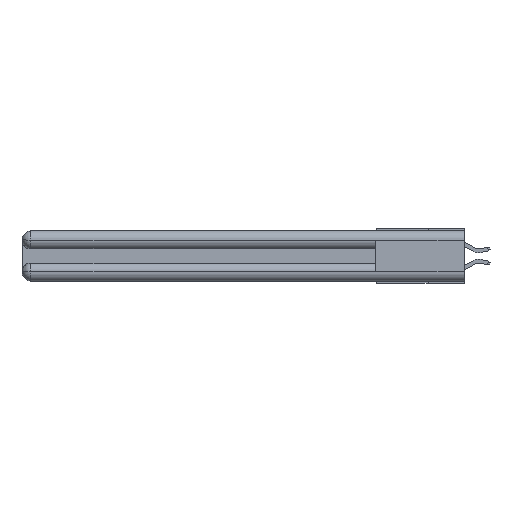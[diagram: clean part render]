
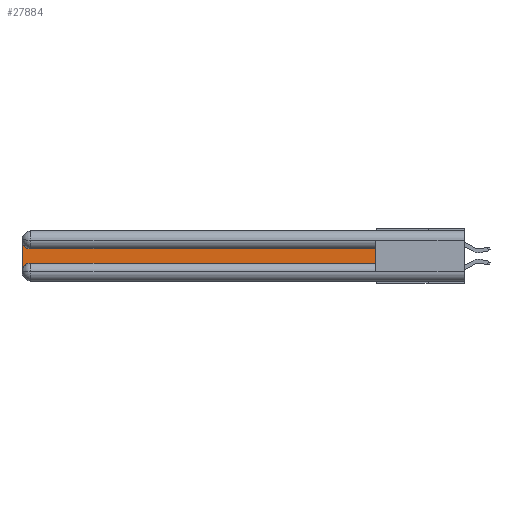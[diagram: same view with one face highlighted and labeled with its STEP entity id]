
A CAD part, left-side view. The second image highlights one B-rep face of the part: STEP entity #27884.
In plain terms, the highlighted planar face has unit normal (-1, 0, 0).
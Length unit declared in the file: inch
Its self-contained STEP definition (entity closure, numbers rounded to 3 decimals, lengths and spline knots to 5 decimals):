
#1772 = DIRECTION ( 'NONE',  ( 0., 0., 1. ) ) ;
#1924 = VERTEX_POINT ( 'NONE', #27431 ) ;
#1940 = VECTOR ( 'NONE', #27641, 39.37008 ) ;
#1979 = CARTESIAN_POINT ( 'NONE',  ( 0.075, 2.94, -0.0625 ) ) ;
#2210 = CARTESIAN_POINT ( 'NONE',  ( 0.075, 2.94, -0.2775 ) ) ;
#2376 = LINE ( 'NONE', #8581, #26684 ) ;
#2886 = LINE ( 'NONE', #5890, #18569 ) ;
#3226 = PLANE ( 'NONE',  #24979 ) ;
#3554 = EDGE_CURVE ( 'NONE', #15105, #20113, #2376, .T. ) ;
#4357 = DIRECTION ( 'NONE',  ( 0., 0., -1. ) ) ;
#5227 = EDGE_LOOP ( 'NONE', ( #24357, #29130, #21365, #7912, #17228, #21772 ) ) ;
#5320 = CARTESIAN_POINT ( 'NONE',  ( 0.075, 3., -0.1225 ) ) ;
#5786 = AXIS2_PLACEMENT_3D ( 'NONE', #1979, #19069, #4357 ) ;
#5890 = CARTESIAN_POINT ( 'NONE',  ( 0.075, 0.6, -0.1225 ) ) ;
#6630 = CARTESIAN_POINT ( 'NONE',  ( 0.075, 3., -0.0625 ) ) ;
#7912 = ORIENTED_EDGE ( 'NONE', *, *, #29048, .T. ) ;
#8039 = DIRECTION ( 'NONE',  ( 1., 0., 0. ) ) ;
#8581 = CARTESIAN_POINT ( 'NONE',  ( 0.075, 0.6, -0.2175 ) ) ;
#11619 = DIRECTION ( 'NONE',  ( 1., 0., 0. ) ) ;
#11685 = LINE ( 'NONE', #15958, #17305 ) ;
#13332 = CARTESIAN_POINT ( 'NONE',  ( 0.075, 0.6, -0.2175 ) ) ;
#14186 = DIRECTION ( 'NONE',  ( 0., 0., -1. ) ) ;
#14983 = DIRECTION ( 'NONE',  ( 0., 1., 0. ) ) ;
#15105 = VERTEX_POINT ( 'NONE', #16944 ) ;
#15958 = CARTESIAN_POINT ( 'NONE',  ( 0.075, 3., -0.2175 ) ) ;
#16944 = CARTESIAN_POINT ( 'NONE',  ( 0.075, 0.6, -0.2175 ) ) ;
#16957 = CIRCLE ( 'NONE', #27410, 0.06 ) ;
#17053 = CIRCLE ( 'NONE', #5786, 0.06 ) ;
#17228 = ORIENTED_EDGE ( 'NONE', *, *, #23624, .T. ) ;
#17305 = VECTOR ( 'NONE', #14186, 39.37008 ) ;
#17605 = EDGE_CURVE ( 'NONE', #25744, #1924, #11685, .T. ) ;
#17643 = LINE ( 'NONE', #13332, #1940 ) ;
#18398 = FACE_OUTER_BOUND ( 'NONE', #5227, .T. ) ;
#18569 = VECTOR ( 'NONE', #14983, 39.37008 ) ;
#19069 = DIRECTION ( 'NONE',  ( 1., 0., 0. ) ) ;
#20113 = VERTEX_POINT ( 'NONE', #27380 ) ;
#21365 = ORIENTED_EDGE ( 'NONE', *, *, #17605, .T. ) ;
#21772 = ORIENTED_EDGE ( 'NONE', *, *, #3554, .T. ) ;
#23624 = EDGE_CURVE ( 'NONE', #28066, #15105, #17643, .T. ) ;
#24357 = ORIENTED_EDGE ( 'NONE', *, *, #26122, .T. ) ;
#24731 = DIRECTION ( 'NONE',  ( 0., 0., -1. ) ) ;
#24979 = AXIS2_PLACEMENT_3D ( 'NONE', #5320, #8039, #24731 ) ;
#25744 = VERTEX_POINT ( 'NONE', #6630 ) ;
#26122 = EDGE_CURVE ( 'NONE', #20113, #27277, #2886, .T. ) ;
#26325 = DIRECTION ( 'NONE',  ( 0., 0., -1. ) ) ;
#26684 = VECTOR ( 'NONE', #1772, 39.37008 ) ;
#27053 = EDGE_CURVE ( 'NONE', #27277, #25744, #17053, .T. ) ;
#27277 = VERTEX_POINT ( 'NONE', #29222 ) ;
#27380 = CARTESIAN_POINT ( 'NONE',  ( 0.075, 0.6, -0.1225 ) ) ;
#27410 = AXIS2_PLACEMENT_3D ( 'NONE', #2210, #11619, #26325 ) ;
#27431 = CARTESIAN_POINT ( 'NONE',  ( 0.075, 3., -0.2775 ) ) ;
#27641 = DIRECTION ( 'NONE',  ( 0., -1., 0. ) ) ;
#27840 = CARTESIAN_POINT ( 'NONE',  ( 0.075, 2.94, -0.2175 ) ) ;
#27884 = ADVANCED_FACE ( 'NONE', ( #18398 ), #3226, .F. ) ;
#28066 = VERTEX_POINT ( 'NONE', #27840 ) ;
#29048 = EDGE_CURVE ( 'NONE', #1924, #28066, #16957, .T. ) ;
#29130 = ORIENTED_EDGE ( 'NONE', *, *, #27053, .T. ) ;
#29222 = CARTESIAN_POINT ( 'NONE',  ( 0.075, 2.94, -0.1225 ) ) ;
